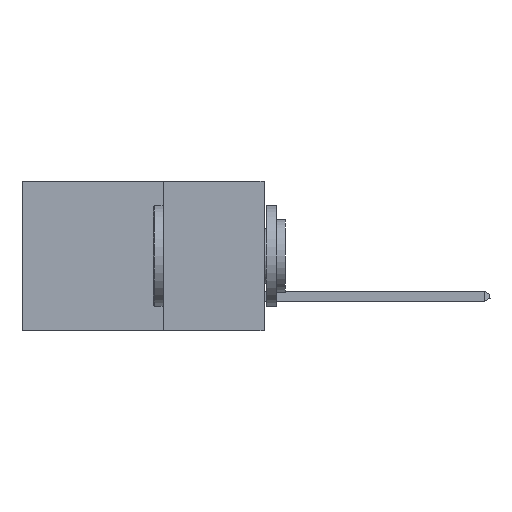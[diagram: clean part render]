
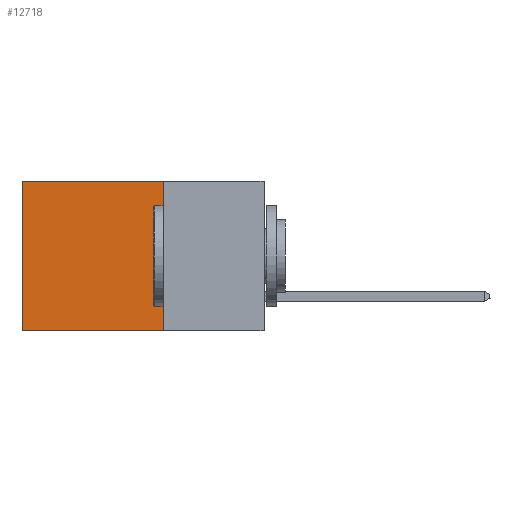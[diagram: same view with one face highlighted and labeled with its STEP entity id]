
A CAD part, left-side view. The second image highlights one B-rep face of the part: STEP entity #12718.
In plain terms, the highlighted planar face has unit normal (-1, 0, 0).
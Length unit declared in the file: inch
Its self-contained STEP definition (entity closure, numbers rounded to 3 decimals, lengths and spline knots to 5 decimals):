
#162 = CARTESIAN_POINT ( 'NONE',  ( 0.298, 0.6, -0.37 ) ) ;
#537 = CARTESIAN_POINT ( 'NONE',  ( 0.298, 0.6, 0. ) ) ;
#1177 = VERTEX_POINT ( 'NONE', #25740 ) ;
#1193 = CARTESIAN_POINT ( 'NONE',  ( 0.298, 0.25, 0. ) ) ;
#2037 = VECTOR ( 'NONE', #24266, 39.37008 ) ;
#3558 = ORIENTED_EDGE ( 'NONE', *, *, #7230, .F. ) ;
#3946 = EDGE_CURVE ( 'NONE', #4929, #8376, #28844, .T. ) ;
#4355 = DIRECTION ( 'NONE',  ( 0., 0., -1. ) ) ;
#4929 = VERTEX_POINT ( 'NONE', #10897 ) ;
#5042 = VECTOR ( 'NONE', #17168, 39.37008 ) ;
#7230 = EDGE_CURVE ( 'NONE', #1177, #18799, #20689, .T. ) ;
#8376 = VERTEX_POINT ( 'NONE', #16842 ) ;
#9555 = LINE ( 'NONE', #12258, #27120 ) ;
#9973 = ORIENTED_EDGE ( 'NONE', *, *, #11765, .T. ) ;
#10897 = CARTESIAN_POINT ( 'NONE',  ( 0.298, 0.25, 0. ) ) ;
#11447 = PLANE ( 'NONE',  #16603 ) ;
#11529 = FACE_OUTER_BOUND ( 'NONE', #14845, .T. ) ;
#11765 = EDGE_CURVE ( 'NONE', #8376, #18799, #26576, .T. ) ;
#12258 = CARTESIAN_POINT ( 'NONE',  ( 0.298, 0.25, 0. ) ) ;
#12511 = DIRECTION ( 'NONE',  ( 0., 0., -1. ) ) ;
#12718 = ADVANCED_FACE ( 'NONE', ( #11529 ), #11447, .F. ) ;
#14661 = ORIENTED_EDGE ( 'NONE', *, *, #3946, .T. ) ;
#14845 = EDGE_LOOP ( 'NONE', ( #9973, #3558, #20191, #14661 ) ) ;
#16603 = AXIS2_PLACEMENT_3D ( 'NONE', #25089, #18424, #4355 ) ;
#16842 = CARTESIAN_POINT ( 'NONE',  ( 0.298, 0.6, 0. ) ) ;
#17168 = DIRECTION ( 'NONE',  ( 0., 1., 0. ) ) ;
#18424 = DIRECTION ( 'NONE',  ( 1., 0., 0. ) ) ;
#18799 = VERTEX_POINT ( 'NONE', #162 ) ;
#20191 = ORIENTED_EDGE ( 'NONE', *, *, #20270, .F. ) ;
#20270 = EDGE_CURVE ( 'NONE', #4929, #1177, #9555, .T. ) ;
#20546 = VECTOR ( 'NONE', #12511, 39.37008 ) ;
#20689 = LINE ( 'NONE', #21997, #2037 ) ;
#21997 = CARTESIAN_POINT ( 'NONE',  ( 0.298, 0.25, -0.37 ) ) ;
#23617 = DIRECTION ( 'NONE',  ( 0., 0., -1. ) ) ;
#24266 = DIRECTION ( 'NONE',  ( 0., 1., 0. ) ) ;
#25089 = CARTESIAN_POINT ( 'NONE',  ( 0.298, 0.25, 0. ) ) ;
#25740 = CARTESIAN_POINT ( 'NONE',  ( 0.298, 0.25, -0.37 ) ) ;
#26576 = LINE ( 'NONE', #537, #20546 ) ;
#27120 = VECTOR ( 'NONE', #23617, 39.37008 ) ;
#28844 = LINE ( 'NONE', #1193, #5042 ) ;
